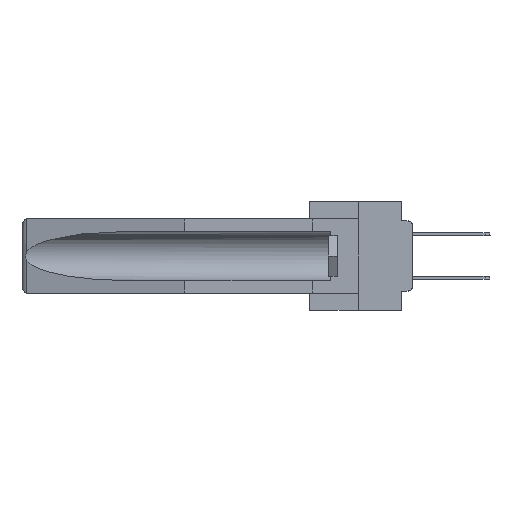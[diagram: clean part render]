
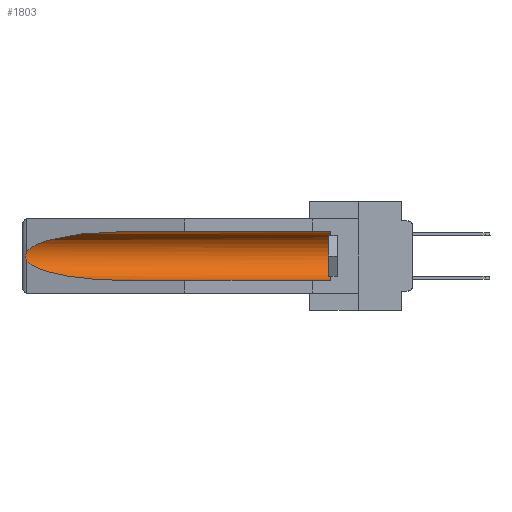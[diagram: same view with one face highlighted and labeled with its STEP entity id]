
A CAD part, left-side view. The second image highlights one B-rep face of the part: STEP entity #1803.
In plain terms, the highlighted cylindrical face has radius 2.857 mm (diameter 5.715 mm), a partial arc.
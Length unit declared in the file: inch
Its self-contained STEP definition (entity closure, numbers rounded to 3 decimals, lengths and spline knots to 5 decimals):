
#20 = CARTESIAN_POINT ( 'NONE',  ( 0.155, 1.07973, -0.059 ) ) ;
#427 = DIRECTION ( 'NONE',  ( 0., -1., 0. ) ) ;
#509 = EDGE_CURVE ( 'NONE', #12196, #16983, #5779, .T. ) ;
#802 = CARTESIAN_POINT ( 'NONE',  ( 0.155, 0.126, -0.284 ) ) ;
#987 = CYLINDRICAL_SURFACE ( 'NONE', #16022, 0.1125 ) ;
#1274 = CARTESIAN_POINT ( 'NONE',  ( 0.155, -0.30754, -0.284 ) ) ;
#1803 = ADVANCED_FACE ( 'NONE', ( #5783 ), #987, .F. ) ;
#2081 = CARTESIAN_POINT ( 'NONE',  ( 0.26597, 1.52961, -0.15275 ) ) ;
#2149 =( BOUNDED_CURVE ( )  B_SPLINE_CURVE ( 3, ( #3183, #19215, #29230, #3521 ),
 .UNSPECIFIED., .F., .F. ) 
 B_SPLINE_CURVE_WITH_KNOTS ( ( 4, 4 ),
 ( 4.71239, 6.08839 ),
 .UNSPECIFIED. ) 
 CURVE ( )  GEOMETRIC_REPRESENTATION_ITEM ( )  RATIONAL_B_SPLINE_CURVE ( ( 1., 0.848, 0.848, 1. ) ) 
 REPRESENTATION_ITEM ( '' )  );
#2178 = CARTESIAN_POINT ( 'NONE',  ( 0.155, 0.126, -0.059 ) ) ;
#3183 = CARTESIAN_POINT ( 'NONE',  ( 0.155, 1.07973, -0.059 ) ) ;
#3277 = VERTEX_POINT ( 'NONE', #2178 ) ;
#3521 = CARTESIAN_POINT ( 'NONE',  ( 0.26537, 1.52718, -0.14972 ) ) ;
#3524 = ORIENTED_EDGE ( 'NONE', *, *, #12112, .T. ) ;
#5232 = B_SPLINE_CURVE_WITH_KNOTS ( 'NONE', 3,
 ( #32549, #2081, #22879, #33237, #32732, #23552, #25922, #23716, #23051, #12823 ),
 .UNSPECIFIED., .F., .F.,
 ( 4, 2, 2, 2, 4 ),
 ( 0., 0.00029, 0.00058, 0.00087, 0.00117 ),
 .UNSPECIFIED. ) ;
#5779 = LINE ( 'NONE', #1274, #14748 ) ;
#5783 = FACE_OUTER_BOUND ( 'NONE', #18840, .T. ) ;
#7033 = CARTESIAN_POINT ( 'NONE',  ( 0.26537, 1.52718, -0.14972 ) ) ;
#7361 = EDGE_CURVE ( 'NONE', #3277, #32662, #14240, .T. ) ;
#8404 = EDGE_CURVE ( 'NONE', #26766, #28698, #5232, .T. ) ;
#8660 = CARTESIAN_POINT ( 'NONE',  ( 0.26537, 1.52718, -0.19328 ) ) ;
#8894 = CIRCLE ( 'NONE', #14868, 0.1125 ) ;
#11684 = CARTESIAN_POINT ( 'NONE',  ( 0.155, -0.30754, -0.059 ) ) ;
#12112 = EDGE_CURVE ( 'NONE', #28698, #16983, #18482, .T. ) ;
#12196 = VERTEX_POINT ( 'NONE', #802 ) ;
#12823 = CARTESIAN_POINT ( 'NONE',  ( 0.26537, 1.52718, -0.19328 ) ) ;
#14079 = ORIENTED_EDGE ( 'NONE', *, *, #22360, .T. ) ;
#14240 = LINE ( 'NONE', #11684, #22187 ) ;
#14748 = VECTOR ( 'NONE', #32424, 39.37008 ) ;
#14868 = AXIS2_PLACEMENT_3D ( 'NONE', #26342, #427, #23453 ) ;
#15102 = CARTESIAN_POINT ( 'NONE',  ( 0.26537, 1.52718, -0.19328 ) ) ;
#16022 = AXIS2_PLACEMENT_3D ( 'NONE', #31985, #16351, #16185 ) ;
#16185 = DIRECTION ( 'NONE',  ( 0., 0., 1. ) ) ;
#16351 = DIRECTION ( 'NONE',  ( 0., 1., 0. ) ) ;
#16983 = VERTEX_POINT ( 'NONE', #21575 ) ;
#18482 =( BOUNDED_CURVE ( )  B_SPLINE_CURVE ( 3, ( #8660, #18720, #18888, #32127 ),
 .UNSPECIFIED., .F., .F. ) 
 B_SPLINE_CURVE_WITH_KNOTS ( ( 4, 4 ),
 ( 0.1948, 1.5708 ),
 .UNSPECIFIED. ) 
 CURVE ( )  GEOMETRIC_REPRESENTATION_ITEM ( )  RATIONAL_B_SPLINE_CURVE ( ( 1., 0.848, 0.848, 1. ) ) 
 REPRESENTATION_ITEM ( '' )  );
#18720 = CARTESIAN_POINT ( 'NONE',  ( 0.25451, 1.48313, -0.24835 ) ) ;
#18840 = EDGE_LOOP ( 'NONE', ( #14079, #31522, #3524, #27218, #26394, #21977 ) ) ;
#18888 = CARTESIAN_POINT ( 'NONE',  ( 0.21114, 1.30732, -0.284 ) ) ;
#19215 = CARTESIAN_POINT ( 'NONE',  ( 0.21114, 1.30732, -0.059 ) ) ;
#19624 = EDGE_CURVE ( 'NONE', #12196, #3277, #8894, .T. ) ;
#21575 = CARTESIAN_POINT ( 'NONE',  ( 0.155, 1.07973, -0.284 ) ) ;
#21977 = ORIENTED_EDGE ( 'NONE', *, *, #7361, .T. ) ;
#22187 = VECTOR ( 'NONE', #32418, 39.37008 ) ;
#22360 = EDGE_CURVE ( 'NONE', #32662, #26766, #2149, .T. ) ;
#22879 = CARTESIAN_POINT ( 'NONE',  ( 0.26654, 1.53092, -0.15636 ) ) ;
#23051 = CARTESIAN_POINT ( 'NONE',  ( 0.26597, 1.5296, -0.19026 ) ) ;
#23453 = DIRECTION ( 'NONE',  ( 0., 0., 1. ) ) ;
#23552 = CARTESIAN_POINT ( 'NONE',  ( 0.2675, 1.53308, -0.17534 ) ) ;
#23716 = CARTESIAN_POINT ( 'NONE',  ( 0.26655, 1.53094, -0.18657 ) ) ;
#25922 = CARTESIAN_POINT ( 'NONE',  ( 0.2673, 1.53269, -0.17917 ) ) ;
#26342 = CARTESIAN_POINT ( 'NONE',  ( 0.155, 0.126, -0.1715 ) ) ;
#26394 = ORIENTED_EDGE ( 'NONE', *, *, #19624, .T. ) ;
#26766 = VERTEX_POINT ( 'NONE', #7033 ) ;
#27218 = ORIENTED_EDGE ( 'NONE', *, *, #509, .F. ) ;
#28698 = VERTEX_POINT ( 'NONE', #15102 ) ;
#29230 = CARTESIAN_POINT ( 'NONE',  ( 0.25451, 1.48313, -0.09465 ) ) ;
#31522 = ORIENTED_EDGE ( 'NONE', *, *, #8404, .T. ) ;
#31985 = CARTESIAN_POINT ( 'NONE',  ( 0.155, -0.30754, -0.1715 ) ) ;
#32127 = CARTESIAN_POINT ( 'NONE',  ( 0.155, 1.07973, -0.284 ) ) ;
#32418 = DIRECTION ( 'NONE',  ( 0., 1., 0. ) ) ;
#32424 = DIRECTION ( 'NONE',  ( 0., 1., 0. ) ) ;
#32549 = CARTESIAN_POINT ( 'NONE',  ( 0.26537, 1.52718, -0.14972 ) ) ;
#32662 = VERTEX_POINT ( 'NONE', #20 ) ;
#32732 = CARTESIAN_POINT ( 'NONE',  ( 0.2675, 1.53308, -0.16763 ) ) ;
#33237 = CARTESIAN_POINT ( 'NONE',  ( 0.2673, 1.5327, -0.16383 ) ) ;
